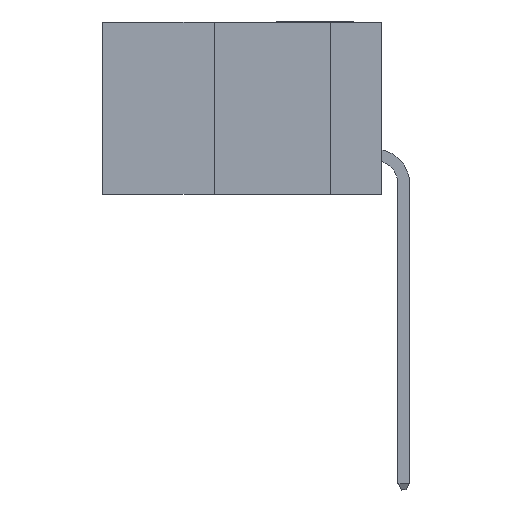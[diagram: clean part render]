
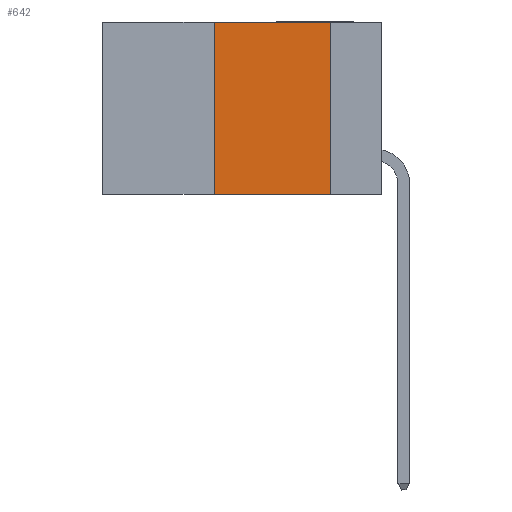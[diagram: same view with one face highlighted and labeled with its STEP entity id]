
A CAD part, left-side view. The second image highlights one B-rep face of the part: STEP entity #642.
In plain terms, the highlighted planar face has unit normal (-1, 0, 0).
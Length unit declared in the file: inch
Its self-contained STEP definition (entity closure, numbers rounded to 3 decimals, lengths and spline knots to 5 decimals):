
#72 = LINE ( 'NONE', #4819, #6910 ) ;
#642 = ADVANCED_FACE ( 'NONE', ( #5540 ), #8335, .F. ) ;
#825 = EDGE_LOOP ( 'NONE', ( #9085, #1988, #5224, #2279 ) ) ;
#857 = LINE ( 'NONE', #7812, #9789 ) ;
#867 = LINE ( 'NONE', #1345, #3180 ) ;
#1262 = EDGE_CURVE ( 'NONE', #2606, #8538, #1611, .T. ) ;
#1345 = CARTESIAN_POINT ( 'NONE',  ( 0., 0.6, -0.37 ) ) ;
#1369 = DIRECTION ( 'NONE',  ( 0., 0., -1. ) ) ;
#1611 = LINE ( 'NONE', #5626, #5492 ) ;
#1850 = EDGE_CURVE ( 'NONE', #2606, #8621, #867, .T. ) ;
#1988 = ORIENTED_EDGE ( 'NONE', *, *, #2395, .F. ) ;
#2016 = CARTESIAN_POINT ( 'NONE',  ( 0., 0.36, 0. ) ) ;
#2079 = DIRECTION ( 'NONE',  ( 0., 0., -1. ) ) ;
#2123 = CARTESIAN_POINT ( 'NONE',  ( 0., 0.11, -0.37 ) ) ;
#2225 = DIRECTION ( 'NONE',  ( 0., -1., 0. ) ) ;
#2279 = ORIENTED_EDGE ( 'NONE', *, *, #1850, .T. ) ;
#2395 = EDGE_CURVE ( 'NONE', #8538, #3464, #857, .T. ) ;
#2606 = VERTEX_POINT ( 'NONE', #8979 ) ;
#3131 = DIRECTION ( 'NONE',  ( 0., -1., 0. ) ) ;
#3180 = VECTOR ( 'NONE', #2225, 39.37008 ) ;
#3464 = VERTEX_POINT ( 'NONE', #8171 ) ;
#3608 = DIRECTION ( 'NONE',  ( 1., 0., 0. ) ) ;
#4819 = CARTESIAN_POINT ( 'NONE',  ( 0., 0.11, 0. ) ) ;
#5132 = AXIS2_PLACEMENT_3D ( 'NONE', #5991, #3608, #1369 ) ;
#5224 = ORIENTED_EDGE ( 'NONE', *, *, #1262, .F. ) ;
#5492 = VECTOR ( 'NONE', #9592, 39.37008 ) ;
#5540 = FACE_OUTER_BOUND ( 'NONE', #825, .T. ) ;
#5626 = CARTESIAN_POINT ( 'NONE',  ( 0., 0.36, 0. ) ) ;
#5991 = CARTESIAN_POINT ( 'NONE',  ( 0., 0.6, 0. ) ) ;
#6211 = EDGE_CURVE ( 'NONE', #3464, #8621, #72, .T. ) ;
#6910 = VECTOR ( 'NONE', #2079, 39.37008 ) ;
#7812 = CARTESIAN_POINT ( 'NONE',  ( 0., 0.6, 0. ) ) ;
#8171 = CARTESIAN_POINT ( 'NONE',  ( 0., 0.11, 0. ) ) ;
#8335 = PLANE ( 'NONE',  #5132 ) ;
#8538 = VERTEX_POINT ( 'NONE', #2016 ) ;
#8621 = VERTEX_POINT ( 'NONE', #2123 ) ;
#8979 = CARTESIAN_POINT ( 'NONE',  ( 0., 0.36, -0.37 ) ) ;
#9085 = ORIENTED_EDGE ( 'NONE', *, *, #6211, .F. ) ;
#9592 = DIRECTION ( 'NONE',  ( 0., 0., 1. ) ) ;
#9789 = VECTOR ( 'NONE', #3131, 39.37008 ) ;
